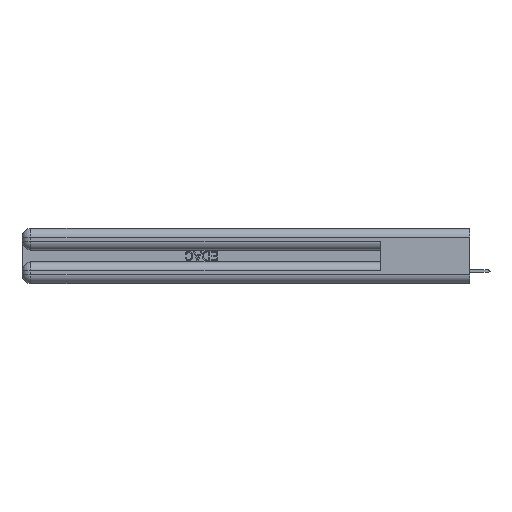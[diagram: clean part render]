
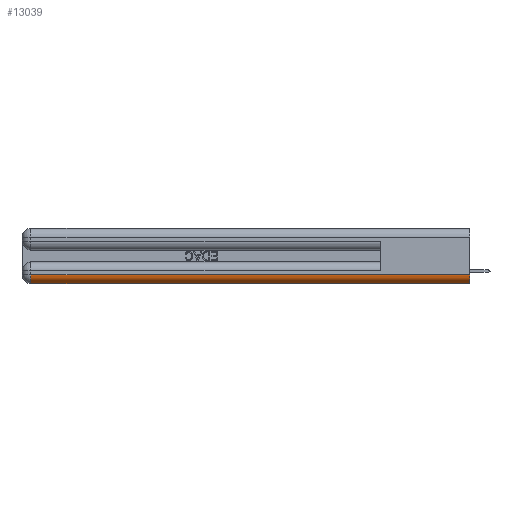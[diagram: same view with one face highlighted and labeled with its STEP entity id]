
A CAD part, left-side view. The second image highlights one B-rep face of the part: STEP entity #13039.
In plain terms, the highlighted cylindrical face has radius 1.524 mm (diameter 3.048 mm), a partial arc.
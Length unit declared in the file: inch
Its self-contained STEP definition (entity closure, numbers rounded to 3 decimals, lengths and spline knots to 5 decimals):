
#105 = CYLINDRICAL_SURFACE ( 'NONE', #45692, 0.06 ) ;
#2431 = EDGE_CURVE ( 'NONE', #21340, #37677, #23249, .T. ) ;
#2643 = DIRECTION ( 'NONE',  ( 0., 1., 0. ) ) ;
#4094 = DIRECTION ( 'NONE',  ( 0., 0., 1. ) ) ;
#4792 = CARTESIAN_POINT ( 'NONE',  ( 0.06, 3., 0. ) ) ;
#6339 = VERTEX_POINT ( 'NONE', #14733 ) ;
#7150 = DIRECTION ( 'NONE',  ( 0., 0., 1. ) ) ;
#10270 = VECTOR ( 'NONE', #29393, 39.37008 ) ;
#10546 = AXIS2_PLACEMENT_3D ( 'NONE', #27796, #2643, #7150 ) ;
#10671 = EDGE_CURVE ( 'NONE', #37677, #47254, #17199, .T. ) ;
#11817 = EDGE_CURVE ( 'NONE', #47254, #6339, #34735, .T. ) ;
#13039 = ADVANCED_FACE ( 'NONE', ( #31361 ), #105, .T. ) ;
#14733 = CARTESIAN_POINT ( 'NONE',  ( 0.06, 0., 0. ) ) ;
#17199 = LINE ( 'NONE', #41316, #10270 ) ;
#17339 = ORIENTED_EDGE ( 'NONE', *, *, #10671, .F. ) ;
#18656 = AXIS2_PLACEMENT_3D ( 'NONE', #28878, #28369, #48731 ) ;
#21340 = VERTEX_POINT ( 'NONE', #29297 ) ;
#23249 = CIRCLE ( 'NONE', #10546, 0.06 ) ;
#24114 = LINE ( 'NONE', #4792, #45291 ) ;
#25849 = ORIENTED_EDGE ( 'NONE', *, *, #11817, .F. ) ;
#27796 = CARTESIAN_POINT ( 'NONE',  ( 0.06, 2.94, 0.06 ) ) ;
#28360 = DIRECTION ( 'NONE',  ( 0., 1., 0. ) ) ;
#28369 = DIRECTION ( 'NONE',  ( 0., -1., 0. ) ) ;
#28878 = CARTESIAN_POINT ( 'NONE',  ( 0.06, 0., 0.06 ) ) ;
#29297 = CARTESIAN_POINT ( 'NONE',  ( 0.06, 2.94, 0. ) ) ;
#29393 = DIRECTION ( 'NONE',  ( 0., -1., 0. ) ) ;
#30982 = EDGE_CURVE ( 'NONE', #6339, #21340, #24114, .T. ) ;
#31301 = CARTESIAN_POINT ( 'NONE',  ( 0., 2.94, 0.06 ) ) ;
#31361 = FACE_OUTER_BOUND ( 'NONE', #36055, .T. ) ;
#34735 = CIRCLE ( 'NONE', #18656, 0.06 ) ;
#36055 = EDGE_LOOP ( 'NONE', ( #25849, #17339, #41511, #38529 ) ) ;
#37313 = CARTESIAN_POINT ( 'NONE',  ( 0., 0., 0.06 ) ) ;
#37677 = VERTEX_POINT ( 'NONE', #31301 ) ;
#38529 = ORIENTED_EDGE ( 'NONE', *, *, #30982, .F. ) ;
#39826 = CARTESIAN_POINT ( 'NONE',  ( 0.06, 0., 0.06 ) ) ;
#40360 = DIRECTION ( 'NONE',  ( 0., 1., 0. ) ) ;
#41316 = CARTESIAN_POINT ( 'NONE',  ( 0., 0., 0.06 ) ) ;
#41511 = ORIENTED_EDGE ( 'NONE', *, *, #2431, .F. ) ;
#45291 = VECTOR ( 'NONE', #28360, 39.37008 ) ;
#45692 = AXIS2_PLACEMENT_3D ( 'NONE', #39826, #40360, #4094 ) ;
#47254 = VERTEX_POINT ( 'NONE', #37313 ) ;
#48731 = DIRECTION ( 'NONE',  ( 0., 0., 1. ) ) ;
